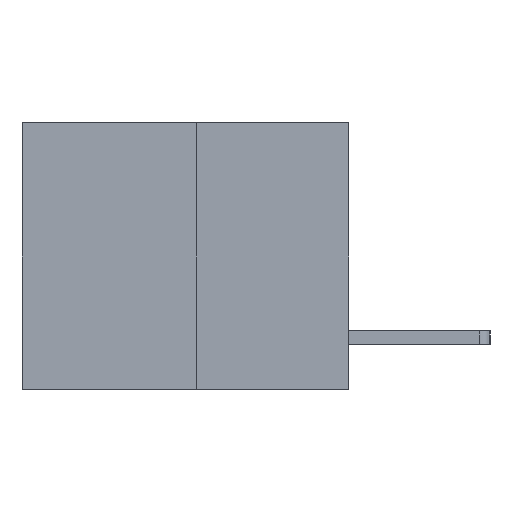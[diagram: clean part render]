
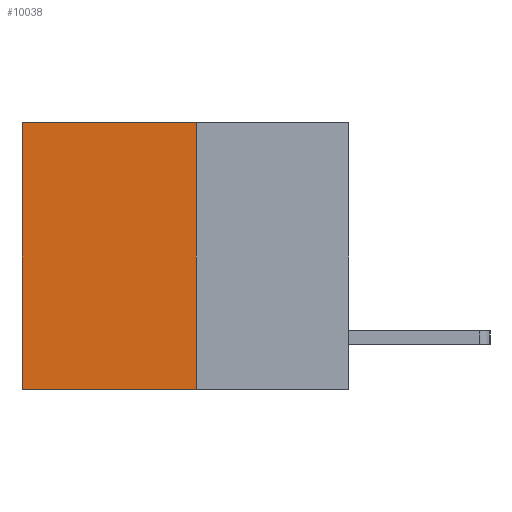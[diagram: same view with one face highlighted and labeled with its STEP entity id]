
A CAD part, left-side view. The second image highlights one B-rep face of the part: STEP entity #10038.
In plain terms, the highlighted planar face has unit normal (-1, 0, 0).
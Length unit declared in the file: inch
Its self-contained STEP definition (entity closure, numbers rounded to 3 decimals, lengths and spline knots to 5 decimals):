
#565 = DIRECTION ( 'NONE',  ( 0., 1., 0. ) ) ;
#693 = VERTEX_POINT ( 'NONE', #10581 ) ;
#887 = DIRECTION ( 'NONE',  ( 1., 0., 0. ) ) ;
#959 = DIRECTION ( 'NONE',  ( 0., 0., -1. ) ) ;
#1106 = CARTESIAN_POINT ( 'NONE',  ( 0.3165, 0.6, -0.49 ) ) ;
#1260 = CARTESIAN_POINT ( 'NONE',  ( 0.3165, 0.6, -0.49 ) ) ;
#1481 = LINE ( 'NONE', #7042, #2729 ) ;
#1664 = DIRECTION ( 'NONE',  ( 0., 1., 0. ) ) ;
#2238 = EDGE_CURVE ( 'NONE', #693, #10674, #8042, .T. ) ;
#2388 = EDGE_LOOP ( 'NONE', ( #3079, #9472, #8791, #3068 ) ) ;
#2573 = CARTESIAN_POINT ( 'NONE',  ( 0.3165, 0.28, -0.49 ) ) ;
#2729 = VECTOR ( 'NONE', #1664, 39.37008 ) ;
#3068 = ORIENTED_EDGE ( 'NONE', *, *, #2238, .T. ) ;
#3079 = ORIENTED_EDGE ( 'NONE', *, *, #8766, .T. ) ;
#3788 = DIRECTION ( 'NONE',  ( 0., 0., -1. ) ) ;
#4437 = CARTESIAN_POINT ( 'NONE',  ( 0.3165, 0.28, -0.49 ) ) ;
#4793 = VECTOR ( 'NONE', #565, 39.37008 ) ;
#4862 = LINE ( 'NONE', #1106, #6970 ) ;
#6118 = VERTEX_POINT ( 'NONE', #6721 ) ;
#6188 = LINE ( 'NONE', #2573, #10985 ) ;
#6721 = CARTESIAN_POINT ( 'NONE',  ( 0.3165, 0.28, -0.49 ) ) ;
#6904 = CARTESIAN_POINT ( 'NONE',  ( 0.3165, 0.6, 0. ) ) ;
#6933 = FACE_OUTER_BOUND ( 'NONE', #2388, .T. ) ;
#6970 = VECTOR ( 'NONE', #3788, 39.37008 ) ;
#6986 = EDGE_CURVE ( 'NONE', #6118, #10487, #1481, .T. ) ;
#7042 = CARTESIAN_POINT ( 'NONE',  ( 0.3165, 0.28, -0.49 ) ) ;
#8042 = LINE ( 'NONE', #8456, #4793 ) ;
#8456 = CARTESIAN_POINT ( 'NONE',  ( 0.3165, 0.28, 0. ) ) ;
#8766 = EDGE_CURVE ( 'NONE', #10674, #10487, #4862, .T. ) ;
#8775 = AXIS2_PLACEMENT_3D ( 'NONE', #4437, #887, #959 ) ;
#8791 = ORIENTED_EDGE ( 'NONE', *, *, #11346, .F. ) ;
#9472 = ORIENTED_EDGE ( 'NONE', *, *, #6986, .F. ) ;
#9963 = PLANE ( 'NONE',  #8775 ) ;
#10038 = ADVANCED_FACE ( 'NONE', ( #6933 ), #9963, .F. ) ;
#10052 = DIRECTION ( 'NONE',  ( 0., 0., -1. ) ) ;
#10487 = VERTEX_POINT ( 'NONE', #1260 ) ;
#10581 = CARTESIAN_POINT ( 'NONE',  ( 0.3165, 0.28, 0. ) ) ;
#10674 = VERTEX_POINT ( 'NONE', #6904 ) ;
#10985 = VECTOR ( 'NONE', #10052, 39.37008 ) ;
#11346 = EDGE_CURVE ( 'NONE', #693, #6118, #6188, .T. ) ;
